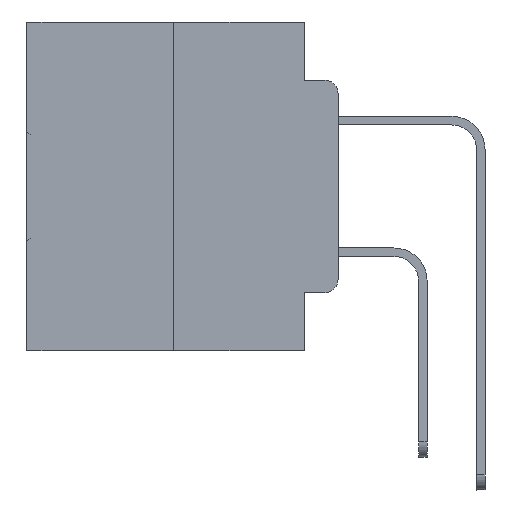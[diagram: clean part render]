
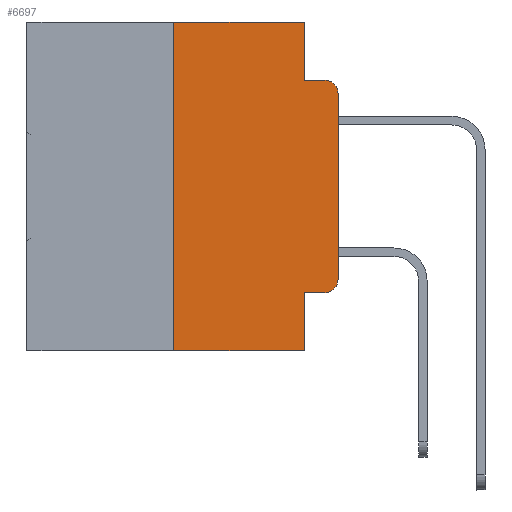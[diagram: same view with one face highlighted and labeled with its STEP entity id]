
A CAD part, left-side view. The second image highlights one B-rep face of the part: STEP entity #6697.
In plain terms, the highlighted planar face has unit normal (-1, 0, 0).
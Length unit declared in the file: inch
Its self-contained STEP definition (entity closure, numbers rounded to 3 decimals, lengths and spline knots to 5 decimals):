
#494 = ORIENTED_EDGE ( 'NONE', *, *, #15224, .T. ) ;
#784 = DIRECTION ( 'NONE',  ( 0., -1., 0. ) ) ;
#1024 = DIRECTION ( 'NONE',  ( 0., 0., -1. ) ) ;
#1710 = DIRECTION ( 'NONE',  ( -1., 0., 0. ) ) ;
#2247 = VERTEX_POINT ( 'NONE', #23480 ) ;
#2336 = EDGE_LOOP ( 'NONE', ( #494, #26043, #3435, #21251, #31197, #20122, #32454, #11632, #22621, #24630 ) ) ;
#2824 = LINE ( 'NONE', #31401, #15884 ) ;
#3006 = EDGE_CURVE ( 'NONE', #9358, #10227, #23870, .T. ) ;
#3094 = LINE ( 'NONE', #17101, #22120 ) ;
#3409 = CARTESIAN_POINT ( 'NONE',  ( 0., 0.473, -0.5 ) ) ;
#3435 = ORIENTED_EDGE ( 'NONE', *, *, #8225, .F. ) ;
#3791 = CARTESIAN_POINT ( 'NONE',  ( 0., 0.051, -0.5 ) ) ;
#3990 = LINE ( 'NONE', #27516, #8409 ) ;
#4843 = CARTESIAN_POINT ( 'NONE',  ( 0., 0., -0.1085 ) ) ;
#6035 = DIRECTION ( 'NONE',  ( 0., -1., 0. ) ) ;
#6518 = EDGE_CURVE ( 'NONE', #17617, #2247, #29553, .T. ) ;
#6697 = ADVANCED_FACE ( 'NONE', ( #29131 ), #27608, .F. ) ;
#7465 = CARTESIAN_POINT ( 'NONE',  ( 0., 0.02, -0.0885 ) ) ;
#7533 = VERTEX_POINT ( 'NONE', #13567 ) ;
#7654 = VERTEX_POINT ( 'NONE', #3791 ) ;
#8225 = EDGE_CURVE ( 'NONE', #2247, #26474, #9320, .T. ) ;
#8409 = VECTOR ( 'NONE', #30097, 39.37008 ) ;
#8920 = DIRECTION ( 'NONE',  ( 0., 0., -1. ) ) ;
#9320 = LINE ( 'NONE', #21505, #22276 ) ;
#9358 = VERTEX_POINT ( 'NONE', #25795 ) ;
#10227 = VERTEX_POINT ( 'NONE', #29660 ) ;
#11632 = ORIENTED_EDGE ( 'NONE', *, *, #32936, .F. ) ;
#12226 = DIRECTION ( 'NONE',  ( 1., 0., 0. ) ) ;
#12513 = VERTEX_POINT ( 'NONE', #13333 ) ;
#13125 = AXIS2_PLACEMENT_3D ( 'NONE', #17366, #1710, #19950 ) ;
#13333 = CARTESIAN_POINT ( 'NONE',  ( 0., 0.02, -0.4115 ) ) ;
#13483 = EDGE_CURVE ( 'NONE', #18120, #26474, #25032, .T. ) ;
#13567 = CARTESIAN_POINT ( 'NONE',  ( 0., 0., -0.3915 ) ) ;
#14119 = CARTESIAN_POINT ( 'NONE',  ( 0., 0.051, 0. ) ) ;
#14136 = LINE ( 'NONE', #31379, #25354 ) ;
#15224 = EDGE_CURVE ( 'NONE', #7533, #18120, #3094, .T. ) ;
#15884 = VECTOR ( 'NONE', #18738, 39.37008 ) ;
#16716 = DIRECTION ( 'NONE',  ( -1., 0., 0. ) ) ;
#17101 = CARTESIAN_POINT ( 'NONE',  ( 0., 0., 0. ) ) ;
#17137 = AXIS2_PLACEMENT_3D ( 'NONE', #31956, #16716, #1024 ) ;
#17366 = CARTESIAN_POINT ( 'NONE',  ( 0., 0.02, -0.1085 ) ) ;
#17617 = VERTEX_POINT ( 'NONE', #14119 ) ;
#18120 = VERTEX_POINT ( 'NONE', #4843 ) ;
#18738 = DIRECTION ( 'NONE',  ( 0., 0., -1. ) ) ;
#19278 = CARTESIAN_POINT ( 'NONE',  ( 0., 0.051, 0. ) ) ;
#19369 = CARTESIAN_POINT ( 'NONE',  ( 0., 0.25, 0. ) ) ;
#19672 = DIRECTION ( 'NONE',  ( 0., 0., 1. ) ) ;
#19950 = DIRECTION ( 'NONE',  ( 0., 0., -1. ) ) ;
#20122 = ORIENTED_EDGE ( 'NONE', *, *, #3006, .F. ) ;
#21251 = ORIENTED_EDGE ( 'NONE', *, *, #6518, .F. ) ;
#21505 = CARTESIAN_POINT ( 'NONE',  ( 0., 0.051, -0.0885 ) ) ;
#22120 = VECTOR ( 'NONE', #19672, 39.37008 ) ;
#22276 = VECTOR ( 'NONE', #784, 39.37008 ) ;
#22449 = DIRECTION ( 'NONE',  ( 0., 0., 1. ) ) ;
#22621 = ORIENTED_EDGE ( 'NONE', *, *, #29597, .T. ) ;
#23480 = CARTESIAN_POINT ( 'NONE',  ( 0., 0.051, -0.0885 ) ) ;
#23870 = LINE ( 'NONE', #19369, #29893 ) ;
#24245 = EDGE_CURVE ( 'NONE', #9358, #7654, #31438, .T. ) ;
#24630 = ORIENTED_EDGE ( 'NONE', *, *, #26162, .T. ) ;
#25032 = CIRCLE ( 'NONE', #13125, 0.02 ) ;
#25354 = VECTOR ( 'NONE', #28958, 39.37008 ) ;
#25558 = VERTEX_POINT ( 'NONE', #31776 ) ;
#25669 = AXIS2_PLACEMENT_3D ( 'NONE', #27506, #12226, #30183 ) ;
#25795 = CARTESIAN_POINT ( 'NONE',  ( 0., 0.25, -0.5 ) ) ;
#26043 = ORIENTED_EDGE ( 'NONE', *, *, #13483, .T. ) ;
#26162 = EDGE_CURVE ( 'NONE', #12513, #7533, #30032, .T. ) ;
#26474 = VERTEX_POINT ( 'NONE', #7465 ) ;
#27506 = CARTESIAN_POINT ( 'NONE',  ( 0., 0.473, 0. ) ) ;
#27516 = CARTESIAN_POINT ( 'NONE',  ( 0., 0.473, 0. ) ) ;
#27608 = PLANE ( 'NONE',  #25669 ) ;
#28749 = VECTOR ( 'NONE', #8920, 39.37008 ) ;
#28958 = DIRECTION ( 'NONE',  ( 0., -1., 0. ) ) ;
#29131 = FACE_OUTER_BOUND ( 'NONE', #2336, .T. ) ;
#29197 = EDGE_CURVE ( 'NONE', #10227, #17617, #3990, .T. ) ;
#29553 = LINE ( 'NONE', #19278, #28749 ) ;
#29597 = EDGE_CURVE ( 'NONE', #25558, #12513, #14136, .T. ) ;
#29660 = CARTESIAN_POINT ( 'NONE',  ( 0., 0.25, 0. ) ) ;
#29893 = VECTOR ( 'NONE', #22449, 39.37008 ) ;
#30032 = CIRCLE ( 'NONE', #17137, 0.02 ) ;
#30097 = DIRECTION ( 'NONE',  ( 0., -1., 0. ) ) ;
#30183 = DIRECTION ( 'NONE',  ( 0., 0., -1. ) ) ;
#30652 = VECTOR ( 'NONE', #6035, 39.37008 ) ;
#31197 = ORIENTED_EDGE ( 'NONE', *, *, #29197, .F. ) ;
#31379 = CARTESIAN_POINT ( 'NONE',  ( 0., 0.051, -0.4115 ) ) ;
#31401 = CARTESIAN_POINT ( 'NONE',  ( 0., 0.051, 0. ) ) ;
#31438 = LINE ( 'NONE', #3409, #30652 ) ;
#31776 = CARTESIAN_POINT ( 'NONE',  ( 0., 0.051, -0.4115 ) ) ;
#31956 = CARTESIAN_POINT ( 'NONE',  ( 0., 0.02, -0.3915 ) ) ;
#32454 = ORIENTED_EDGE ( 'NONE', *, *, #24245, .T. ) ;
#32936 = EDGE_CURVE ( 'NONE', #25558, #7654, #2824, .T. ) ;
